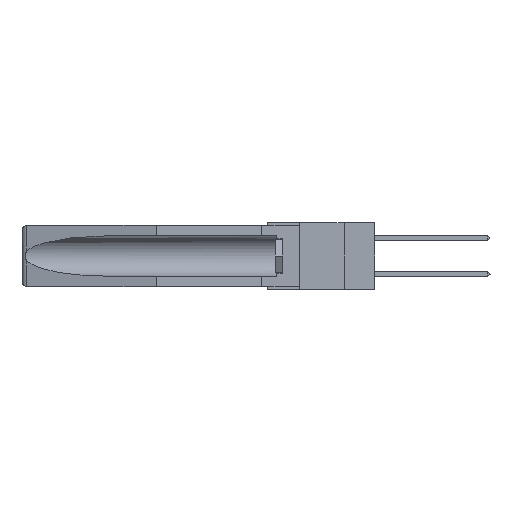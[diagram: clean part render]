
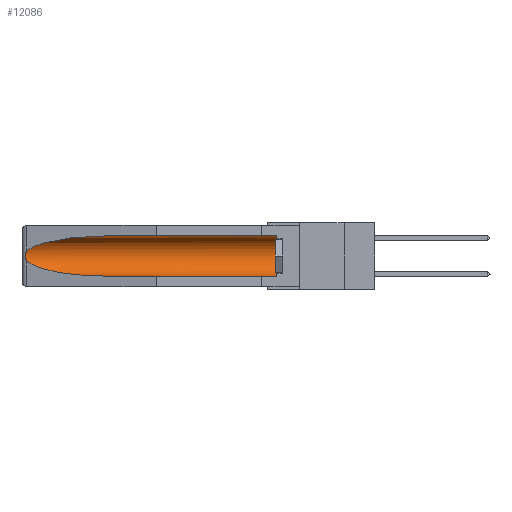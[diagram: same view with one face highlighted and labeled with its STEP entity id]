
A CAD part, left-side view. The second image highlights one B-rep face of the part: STEP entity #12086.
In plain terms, the highlighted cylindrical face has radius 2.857 mm (diameter 5.715 mm), a partial arc.
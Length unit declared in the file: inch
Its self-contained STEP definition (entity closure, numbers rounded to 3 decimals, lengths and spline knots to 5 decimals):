
#814 = CARTESIAN_POINT ( 'NONE',  ( 0.25451, 1.48313, -0.09465 ) ) ;
#1024 = ORIENTED_EDGE ( 'NONE', *, *, #18691, .T. ) ;
#1229 = CARTESIAN_POINT ( 'NONE',  ( 0.26537, 1.52718, -0.14972 ) ) ;
#1497 = CARTESIAN_POINT ( 'NONE',  ( 0.2675, 1.53308, -0.16763 ) ) ;
#1762 = DIRECTION ( 'NONE',  ( 0., 0., 1. ) ) ;
#1768 = EDGE_LOOP ( 'NONE', ( #14116, #1024, #20560, #18288, #7336, #4319 ) ) ;
#1919 = CARTESIAN_POINT ( 'NONE',  ( 0.155, 0.126, -0.1715 ) ) ;
#2456 = VERTEX_POINT ( 'NONE', #8720 ) ;
#2992 = EDGE_CURVE ( 'NONE', #13199, #4262, #4542, .T. ) ;
#3073 =( BOUNDED_CURVE ( )  B_SPLINE_CURVE ( 3, ( #21170, #23036, #11783, #17496 ),
 .UNSPECIFIED., .F., .F. ) 
 B_SPLINE_CURVE_WITH_KNOTS ( ( 4, 4 ),
 ( 0.1948, 1.5708 ),
 .UNSPECIFIED. ) 
 CURVE ( )  GEOMETRIC_REPRESENTATION_ITEM ( )  RATIONAL_B_SPLINE_CURVE ( ( 1., 0.848, 0.848, 1. ) ) 
 REPRESENTATION_ITEM ( '' )  );
#3926 = CARTESIAN_POINT ( 'NONE',  ( 0.26597, 1.5296, -0.19026 ) ) ;
#4147 = CIRCLE ( 'NONE', #11819, 0.1125 ) ;
#4262 = VERTEX_POINT ( 'NONE', #8220 ) ;
#4319 = ORIENTED_EDGE ( 'NONE', *, *, #15536, .T. ) ;
#4542 = LINE ( 'NONE', #6374, #8362 ) ;
#4970 = CARTESIAN_POINT ( 'NONE',  ( 0.26537, 1.52718, -0.19328 ) ) ;
#5585 = CARTESIAN_POINT ( 'NONE',  ( 0.26654, 1.53092, -0.15636 ) ) ;
#5608 =( BOUNDED_CURVE ( )  B_SPLINE_CURVE ( 3, ( #23221, #15627, #814, #15792 ),
 .UNSPECIFIED., .F., .F. ) 
 B_SPLINE_CURVE_WITH_KNOTS ( ( 4, 4 ),
 ( 4.71239, 6.08839 ),
 .UNSPECIFIED. ) 
 CURVE ( )  GEOMETRIC_REPRESENTATION_ITEM ( )  RATIONAL_B_SPLINE_CURVE ( ( 1., 0.848, 0.848, 1. ) ) 
 REPRESENTATION_ITEM ( '' )  );
#6374 = CARTESIAN_POINT ( 'NONE',  ( 0.155, -0.30754, -0.284 ) ) ;
#6622 = CARTESIAN_POINT ( 'NONE',  ( 0.155, -0.30754, -0.1715 ) ) ;
#7336 = ORIENTED_EDGE ( 'NONE', *, *, #22426, .T. ) ;
#7883 = CARTESIAN_POINT ( 'NONE',  ( 0.2675, 1.53308, -0.17534 ) ) ;
#8178 = DIRECTION ( 'NONE',  ( 0., 1., 0. ) ) ;
#8220 = CARTESIAN_POINT ( 'NONE',  ( 0.155, 1.07973, -0.284 ) ) ;
#8362 = VECTOR ( 'NONE', #19475, 39.37008 ) ;
#8367 = VERTEX_POINT ( 'NONE', #9261 ) ;
#8412 = EDGE_CURVE ( 'NONE', #24206, #4262, #3073, .T. ) ;
#8720 = CARTESIAN_POINT ( 'NONE',  ( 0.155, 0.126, -0.059 ) ) ;
#9193 = CYLINDRICAL_SURFACE ( 'NONE', #17807, 0.1125 ) ;
#9261 = CARTESIAN_POINT ( 'NONE',  ( 0.155, 1.07973, -0.059 ) ) ;
#9721 = VERTEX_POINT ( 'NONE', #1229 ) ;
#11430 = VECTOR ( 'NONE', #8178, 39.37008 ) ;
#11783 = CARTESIAN_POINT ( 'NONE',  ( 0.21114, 1.30732, -0.284 ) ) ;
#11819 = AXIS2_PLACEMENT_3D ( 'NONE', #1919, #16997, #1762 ) ;
#12086 = ADVANCED_FACE ( 'NONE', ( #20886 ), #9193, .F. ) ;
#12854 = DIRECTION ( 'NONE',  ( 0., 0., 1. ) ) ;
#13199 = VERTEX_POINT ( 'NONE', #23668 ) ;
#13391 = CARTESIAN_POINT ( 'NONE',  ( 0.26537, 1.52718, -0.19328 ) ) ;
#13999 = DIRECTION ( 'NONE',  ( 0., 1., 0. ) ) ;
#14116 = ORIENTED_EDGE ( 'NONE', *, *, #16371, .T. ) ;
#15536 = EDGE_CURVE ( 'NONE', #2456, #8367, #17579, .T. ) ;
#15627 = CARTESIAN_POINT ( 'NONE',  ( 0.21114, 1.30732, -0.059 ) ) ;
#15792 = CARTESIAN_POINT ( 'NONE',  ( 0.26537, 1.52718, -0.14972 ) ) ;
#16371 = EDGE_CURVE ( 'NONE', #8367, #9721, #5608, .T. ) ;
#16997 = DIRECTION ( 'NONE',  ( 0., -1., 0. ) ) ;
#17496 = CARTESIAN_POINT ( 'NONE',  ( 0.155, 1.07973, -0.284 ) ) ;
#17498 = CARTESIAN_POINT ( 'NONE',  ( 0.155, -0.30754, -0.059 ) ) ;
#17579 = LINE ( 'NONE', #17498, #11430 ) ;
#17807 = AXIS2_PLACEMENT_3D ( 'NONE', #6622, #13999, #12854 ) ;
#18288 = ORIENTED_EDGE ( 'NONE', *, *, #2992, .F. ) ;
#18683 = B_SPLINE_CURVE_WITH_KNOTS ( 'NONE', 3,
 ( #21968, #19932, #5585, #23906, #1497, #7883, #20640, #22593, #3926, #13391 ),
 .UNSPECIFIED., .F., .F.,
 ( 4, 2, 2, 2, 4 ),
 ( 0., 0.00029, 0.00058, 0.00087, 0.00117 ),
 .UNSPECIFIED. ) ;
#18691 = EDGE_CURVE ( 'NONE', #9721, #24206, #18683, .T. ) ;
#19475 = DIRECTION ( 'NONE',  ( 0., 1., 0. ) ) ;
#19932 = CARTESIAN_POINT ( 'NONE',  ( 0.26597, 1.52961, -0.15275 ) ) ;
#20560 = ORIENTED_EDGE ( 'NONE', *, *, #8412, .T. ) ;
#20640 = CARTESIAN_POINT ( 'NONE',  ( 0.2673, 1.53269, -0.17917 ) ) ;
#20886 = FACE_OUTER_BOUND ( 'NONE', #1768, .T. ) ;
#21170 = CARTESIAN_POINT ( 'NONE',  ( 0.26537, 1.52718, -0.19328 ) ) ;
#21968 = CARTESIAN_POINT ( 'NONE',  ( 0.26537, 1.52718, -0.14972 ) ) ;
#22426 = EDGE_CURVE ( 'NONE', #13199, #2456, #4147, .T. ) ;
#22593 = CARTESIAN_POINT ( 'NONE',  ( 0.26655, 1.53094, -0.18657 ) ) ;
#23036 = CARTESIAN_POINT ( 'NONE',  ( 0.25451, 1.48313, -0.24835 ) ) ;
#23221 = CARTESIAN_POINT ( 'NONE',  ( 0.155, 1.07973, -0.059 ) ) ;
#23668 = CARTESIAN_POINT ( 'NONE',  ( 0.155, 0.126, -0.284 ) ) ;
#23906 = CARTESIAN_POINT ( 'NONE',  ( 0.2673, 1.5327, -0.16383 ) ) ;
#24206 = VERTEX_POINT ( 'NONE', #4970 ) ;
